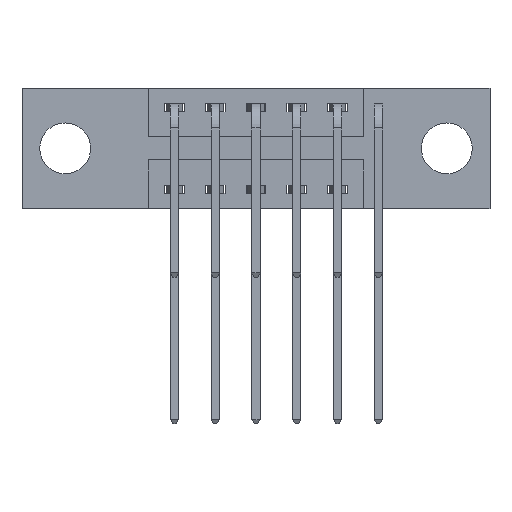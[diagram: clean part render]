
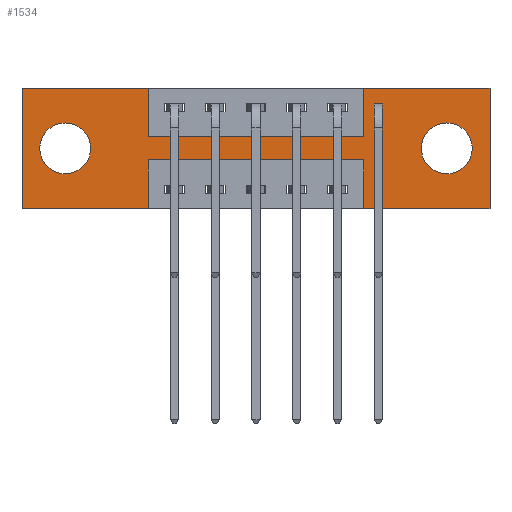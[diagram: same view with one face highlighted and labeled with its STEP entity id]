
A CAD part, front view. The second image highlights one B-rep face of the part: STEP entity #1534.
In plain terms, the highlighted planar face has unit normal (0, -1, 0).
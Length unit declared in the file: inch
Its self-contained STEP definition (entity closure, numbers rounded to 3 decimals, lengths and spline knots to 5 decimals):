
#138 = CARTESIAN_POINT ( 'NONE',  ( 0.3875, 0., -0.22 ) ) ;
#156 = CARTESIAN_POINT ( 'NONE',  ( 0., 0., 0. ) ) ;
#165 = DIRECTION ( 'NONE',  ( 0., 1., 0. ) ) ;
#171 = LINE ( 'NONE', #1088, #6438 ) ;
#283 = CIRCLE ( 'NONE', #10129, 0.078 ) ;
#418 = CARTESIAN_POINT ( 'NONE',  ( 1.0475, 0., 0. ) ) ;
#516 = AXIS2_PLACEMENT_3D ( 'NONE', #6487, #7245, #10470 ) ;
#577 = VECTOR ( 'NONE', #8123, 39.37008 ) ;
#587 = VECTOR ( 'NONE', #3275, 39.37008 ) ;
#643 = ORIENTED_EDGE ( 'NONE', *, *, #4135, .T. ) ;
#658 = CARTESIAN_POINT ( 'NONE',  ( 0.3875, 0., -0.37 ) ) ;
#694 = ORIENTED_EDGE ( 'NONE', *, *, #6518, .F. ) ;
#760 = DIRECTION ( 'NONE',  ( 0., 0., 1. ) ) ;
#931 = CARTESIAN_POINT ( 'NONE',  ( 1.0475, 0., -0.15 ) ) ;
#952 = CARTESIAN_POINT ( 'NONE',  ( 0.3875, 0., 0. ) ) ;
#965 = VERTEX_POINT ( 'NONE', #10442 ) ;
#977 = EDGE_CURVE ( 'NONE', #9709, #6058, #9631, .T. ) ;
#995 = AXIS2_PLACEMENT_3D ( 'NONE', #1792, #3224, #4924 ) ;
#1047 = ORIENTED_EDGE ( 'NONE', *, *, #8367, .F. ) ;
#1088 = CARTESIAN_POINT ( 'NONE',  ( 0., 0., 0. ) ) ;
#1374 = DIRECTION ( 'NONE',  ( 0., 0., 1. ) ) ;
#1433 = CARTESIAN_POINT ( 'NONE',  ( 1.435, 0., 0. ) ) ;
#1494 = DIRECTION ( 'NONE',  ( -1., 0., 0. ) ) ;
#1534 = ADVANCED_FACE ( 'NONE', ( #2579, #3472, #9769 ), #6606, .T. ) ;
#1542 = VERTEX_POINT ( 'NONE', #3422 ) ;
#1792 = CARTESIAN_POINT ( 'NONE',  ( 1.3025, 0., -0.185 ) ) ;
#1818 = ORIENTED_EDGE ( 'NONE', *, *, #4434, .F. ) ;
#1904 = EDGE_CURVE ( 'NONE', #2171, #7689, #283, .T. ) ;
#2171 = VERTEX_POINT ( 'NONE', #7680 ) ;
#2240 = EDGE_CURVE ( 'NONE', #9784, #5267, #10403, .T. ) ;
#2282 = ORIENTED_EDGE ( 'NONE', *, *, #5705, .T. ) ;
#2330 = ORIENTED_EDGE ( 'NONE', *, *, #5818, .F. ) ;
#2335 = CARTESIAN_POINT ( 'NONE',  ( 0.3875, 0., -0.15 ) ) ;
#2394 = DIRECTION ( 'NONE',  ( -1., 0., 0. ) ) ;
#2477 = AXIS2_PLACEMENT_3D ( 'NONE', #5774, #6562, #8960 ) ;
#2579 = FACE_BOUND ( 'NONE', #4880, .T. ) ;
#2791 = CARTESIAN_POINT ( 'NONE',  ( 1.435, 0., -0.37 ) ) ;
#2836 = VERTEX_POINT ( 'NONE', #138 ) ;
#2870 = CARTESIAN_POINT ( 'NONE',  ( 0.3875, 0., -0.15 ) ) ;
#2963 = CARTESIAN_POINT ( 'NONE',  ( 0., 0., -0.37 ) ) ;
#3131 = EDGE_CURVE ( 'NONE', #4255, #1542, #8795, .T. ) ;
#3166 = AXIS2_PLACEMENT_3D ( 'NONE', #4991, #165, #7299 ) ;
#3195 = LINE ( 'NONE', #658, #9484 ) ;
#3213 = CARTESIAN_POINT ( 'NONE',  ( 0.3875, 0., -0.22 ) ) ;
#3224 = DIRECTION ( 'NONE',  ( 0., 1., 0. ) ) ;
#3275 = DIRECTION ( 'NONE',  ( 0., 0., -1. ) ) ;
#3422 = CARTESIAN_POINT ( 'NONE',  ( 1.0475, 0., -0.37 ) ) ;
#3472 = FACE_BOUND ( 'NONE', #10177, .T. ) ;
#3675 = EDGE_CURVE ( 'NONE', #4810, #965, #4851, .T. ) ;
#3726 = CARTESIAN_POINT ( 'NONE',  ( 0.3875, 0., -0.37 ) ) ;
#3755 = DIRECTION ( 'NONE',  ( 0., 0., -1. ) ) ;
#3942 = CARTESIAN_POINT ( 'NONE',  ( 0.1325, 0., -0.107 ) ) ;
#3978 = ORIENTED_EDGE ( 'NONE', *, *, #2240, .F. ) ;
#3998 = VECTOR ( 'NONE', #1494, 39.37008 ) ;
#4032 = CIRCLE ( 'NONE', #995, 0.078 ) ;
#4100 = CARTESIAN_POINT ( 'NONE',  ( 1.0475, 0., -0.22 ) ) ;
#4135 = EDGE_CURVE ( 'NONE', #965, #4810, #4032, .T. ) ;
#4255 = VERTEX_POINT ( 'NONE', #2791 ) ;
#4393 = CARTESIAN_POINT ( 'NONE',  ( 0., 0., -0.37 ) ) ;
#4434 = EDGE_CURVE ( 'NONE', #2836, #9784, #3195, .T. ) ;
#4496 = LINE ( 'NONE', #5186, #7144 ) ;
#4539 = VERTEX_POINT ( 'NONE', #931 ) ;
#4786 = EDGE_LOOP ( 'NONE', ( #1818, #10508, #694, #10526, #10049, #6433, #1047, #10519, #10354, #2330, #6619, #3978 ) ) ;
#4810 = VERTEX_POINT ( 'NONE', #5688 ) ;
#4851 = CIRCLE ( 'NONE', #3166, 0.078 ) ;
#4880 = EDGE_LOOP ( 'NONE', ( #5890, #643 ) ) ;
#4924 = DIRECTION ( 'NONE',  ( 0., 0., -1. ) ) ;
#4967 = LINE ( 'NONE', #7444, #7151 ) ;
#4991 = CARTESIAN_POINT ( 'NONE',  ( 1.3025, 0., -0.185 ) ) ;
#5186 = CARTESIAN_POINT ( 'NONE',  ( 0., 0., 0. ) ) ;
#5234 = VECTOR ( 'NONE', #6112, 39.37008 ) ;
#5244 = CIRCLE ( 'NONE', #516, 0.078 ) ;
#5267 = VERTEX_POINT ( 'NONE', #4393 ) ;
#5298 = VECTOR ( 'NONE', #5956, 39.37008 ) ;
#5612 = EDGE_CURVE ( 'NONE', #6058, #4539, #10191, .T. ) ;
#5688 = CARTESIAN_POINT ( 'NONE',  ( 1.3025, 0., -0.107 ) ) ;
#5705 = EDGE_CURVE ( 'NONE', #7689, #2171, #5244, .T. ) ;
#5717 = CARTESIAN_POINT ( 'NONE',  ( 0.3875, 0., 0. ) ) ;
#5774 = CARTESIAN_POINT ( 'NONE',  ( 0., 0., -0.37 ) ) ;
#5818 = EDGE_CURVE ( 'NONE', #8799, #9709, #171, .T. ) ;
#5881 = DIRECTION ( 'NONE',  ( 0., 0., 1. ) ) ;
#5890 = ORIENTED_EDGE ( 'NONE', *, *, #3675, .T. ) ;
#5956 = DIRECTION ( 'NONE',  ( 1., 0., 0. ) ) ;
#6038 = VERTEX_POINT ( 'NONE', #4100 ) ;
#6058 = VERTEX_POINT ( 'NONE', #2335 ) ;
#6112 = DIRECTION ( 'NONE',  ( 1., 0., 0. ) ) ;
#6261 = EDGE_CURVE ( 'NONE', #5267, #8799, #4496, .T. ) ;
#6290 = EDGE_CURVE ( 'NONE', #7948, #4255, #10220, .T. ) ;
#6433 = ORIENTED_EDGE ( 'NONE', *, *, #7840, .F. ) ;
#6438 = VECTOR ( 'NONE', #9106, 39.37008 ) ;
#6487 = CARTESIAN_POINT ( 'NONE',  ( 0.1325, 0., -0.185 ) ) ;
#6518 = EDGE_CURVE ( 'NONE', #1542, #6038, #4967, .T. ) ;
#6562 = DIRECTION ( 'NONE',  ( 0., -1., 0. ) ) ;
#6606 = PLANE ( 'NONE',  #2477 ) ;
#6619 = ORIENTED_EDGE ( 'NONE', *, *, #6261, .F. ) ;
#6857 = VECTOR ( 'NONE', #1374, 39.37008 ) ;
#7022 = CARTESIAN_POINT ( 'NONE',  ( 0.1325, 0., -0.185 ) ) ;
#7144 = VECTOR ( 'NONE', #7813, 39.37008 ) ;
#7151 = VECTOR ( 'NONE', #5881, 39.37008 ) ;
#7245 = DIRECTION ( 'NONE',  ( 0., 1., 0. ) ) ;
#7299 = DIRECTION ( 'NONE',  ( 0., 0., -1. ) ) ;
#7444 = CARTESIAN_POINT ( 'NONE',  ( 1.0475, 0., -0.37 ) ) ;
#7572 = LINE ( 'NONE', #8462, #5298 ) ;
#7680 = CARTESIAN_POINT ( 'NONE',  ( 0.1325, 0., -0.263 ) ) ;
#7689 = VERTEX_POINT ( 'NONE', #3942 ) ;
#7813 = DIRECTION ( 'NONE',  ( 0., 0., 1. ) ) ;
#7840 = EDGE_CURVE ( 'NONE', #8691, #7948, #7572, .T. ) ;
#7948 = VERTEX_POINT ( 'NONE', #1433 ) ;
#8012 = LINE ( 'NONE', #3213, #577 ) ;
#8123 = DIRECTION ( 'NONE',  ( -1., 0., 0. ) ) ;
#8272 = VECTOR ( 'NONE', #2394, 39.37008 ) ;
#8355 = VECTOR ( 'NONE', #3755, 39.37008 ) ;
#8367 = EDGE_CURVE ( 'NONE', #4539, #8691, #8650, .T. ) ;
#8462 = CARTESIAN_POINT ( 'NONE',  ( 0., 0., 0. ) ) ;
#8560 = EDGE_CURVE ( 'NONE', #6038, #2836, #8012, .T. ) ;
#8629 = DIRECTION ( 'NONE',  ( 0., 1., 0. ) ) ;
#8650 = LINE ( 'NONE', #418, #6857 ) ;
#8691 = VERTEX_POINT ( 'NONE', #9740 ) ;
#8795 = LINE ( 'NONE', #10473, #8272 ) ;
#8799 = VERTEX_POINT ( 'NONE', #156 ) ;
#8960 = DIRECTION ( 'NONE',  ( 0., 0., -1. ) ) ;
#9106 = DIRECTION ( 'NONE',  ( 1., 0., 0. ) ) ;
#9362 = CARTESIAN_POINT ( 'NONE',  ( 1.435, 0., 0. ) ) ;
#9484 = VECTOR ( 'NONE', #9714, 39.37008 ) ;
#9631 = LINE ( 'NONE', #952, #587 ) ;
#9709 = VERTEX_POINT ( 'NONE', #5717 ) ;
#9714 = DIRECTION ( 'NONE',  ( 0., 0., -1. ) ) ;
#9740 = CARTESIAN_POINT ( 'NONE',  ( 1.0475, 0., 0. ) ) ;
#9769 = FACE_OUTER_BOUND ( 'NONE', #4786, .T. ) ;
#9784 = VERTEX_POINT ( 'NONE', #3726 ) ;
#9877 = ORIENTED_EDGE ( 'NONE', *, *, #1904, .T. ) ;
#10049 = ORIENTED_EDGE ( 'NONE', *, *, #6290, .F. ) ;
#10129 = AXIS2_PLACEMENT_3D ( 'NONE', #7022, #8629, #760 ) ;
#10177 = EDGE_LOOP ( 'NONE', ( #2282, #9877 ) ) ;
#10191 = LINE ( 'NONE', #2870, #5234 ) ;
#10220 = LINE ( 'NONE', #9362, #8355 ) ;
#10354 = ORIENTED_EDGE ( 'NONE', *, *, #977, .F. ) ;
#10403 = LINE ( 'NONE', #2963, #3998 ) ;
#10442 = CARTESIAN_POINT ( 'NONE',  ( 1.3025, 0., -0.263 ) ) ;
#10470 = DIRECTION ( 'NONE',  ( 0., 0., 1. ) ) ;
#10473 = CARTESIAN_POINT ( 'NONE',  ( 0., 0., -0.37 ) ) ;
#10508 = ORIENTED_EDGE ( 'NONE', *, *, #8560, .F. ) ;
#10519 = ORIENTED_EDGE ( 'NONE', *, *, #5612, .F. ) ;
#10526 = ORIENTED_EDGE ( 'NONE', *, *, #3131, .F. ) ;
